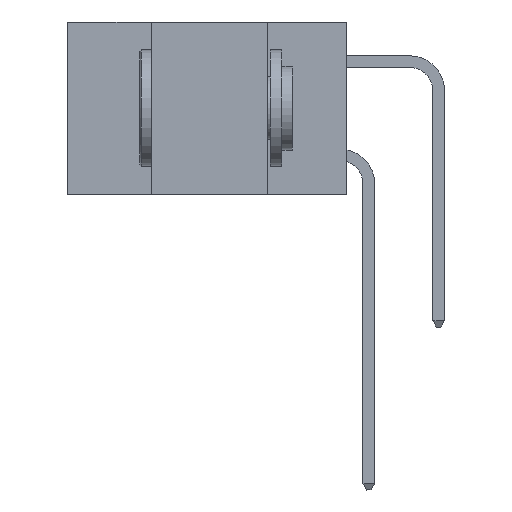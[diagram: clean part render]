
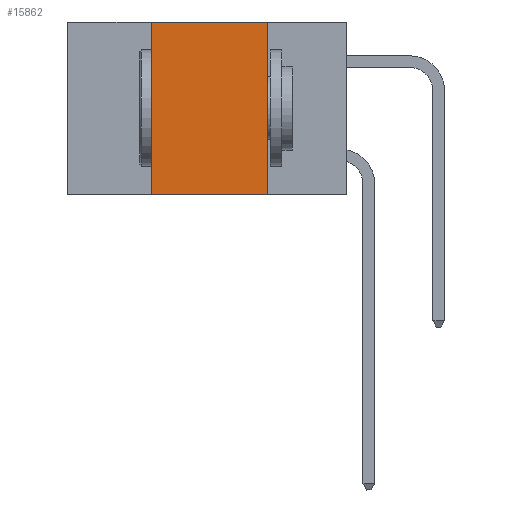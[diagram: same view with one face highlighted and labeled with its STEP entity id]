
A CAD part, left-side view. The second image highlights one B-rep face of the part: STEP entity #15862.
In plain terms, the highlighted planar face has unit normal (-1, 0, 0).
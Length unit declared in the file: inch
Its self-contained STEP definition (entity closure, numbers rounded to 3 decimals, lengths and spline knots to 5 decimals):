
#736 = EDGE_LOOP ( 'NONE', ( #25072, #14019, #37678, #6269 ) ) ;
#1082 = VERTEX_POINT ( 'NONE', #15714 ) ;
#1571 = VERTEX_POINT ( 'NONE', #8951 ) ;
#5653 = PLANE ( 'NONE',  #16178 ) ;
#6269 = ORIENTED_EDGE ( 'NONE', *, *, #40783, .T. ) ;
#6844 = VERTEX_POINT ( 'NONE', #40842 ) ;
#7020 = VECTOR ( 'NONE', #7798, 39.37008 ) ;
#7798 = DIRECTION ( 'NONE',  ( 0., -1., 0. ) ) ;
#8951 = CARTESIAN_POINT ( 'NONE',  ( 0., 0.42, -0.37 ) ) ;
#9311 = DIRECTION ( 'NONE',  ( 0., -1., 0. ) ) ;
#10511 = CARTESIAN_POINT ( 'NONE',  ( 0., 0.6, 0. ) ) ;
#11087 = LINE ( 'NONE', #10511, #7020 ) ;
#11624 = EDGE_CURVE ( 'NONE', #1571, #31572, #41164, .T. ) ;
#14019 = ORIENTED_EDGE ( 'NONE', *, *, #26578, .F. ) ;
#14582 = EDGE_CURVE ( 'NONE', #6844, #1082, #19150, .T. ) ;
#15714 = CARTESIAN_POINT ( 'NONE',  ( 0., 0.17, -0.37 ) ) ;
#15862 = ADVANCED_FACE ( 'NONE', ( #41789 ), #5653, .F. ) ;
#16178 = AXIS2_PLACEMENT_3D ( 'NONE', #28473, #18866, #37911 ) ;
#17213 = LINE ( 'NONE', #19111, #40943 ) ;
#18866 = DIRECTION ( 'NONE',  ( 1., 0., 0. ) ) ;
#19111 = CARTESIAN_POINT ( 'NONE',  ( 0., 0.6, -0.37 ) ) ;
#19150 = LINE ( 'NONE', #24515, #32268 ) ;
#21413 = DIRECTION ( 'NONE',  ( 0., 0., -1. ) ) ;
#23064 = DIRECTION ( 'NONE',  ( 0., 0., 1. ) ) ;
#24515 = CARTESIAN_POINT ( 'NONE',  ( 0., 0.17, 0. ) ) ;
#25072 = ORIENTED_EDGE ( 'NONE', *, *, #14582, .F. ) ;
#26578 = EDGE_CURVE ( 'NONE', #31572, #6844, #11087, .T. ) ;
#26909 = CARTESIAN_POINT ( 'NONE',  ( 0., 0.42, 0. ) ) ;
#28473 = CARTESIAN_POINT ( 'NONE',  ( 0., 0.6, 0. ) ) ;
#31566 = VECTOR ( 'NONE', #23064, 39.37008 ) ;
#31572 = VERTEX_POINT ( 'NONE', #26909 ) ;
#32268 = VECTOR ( 'NONE', #21413, 39.37008 ) ;
#36296 = CARTESIAN_POINT ( 'NONE',  ( 0., 0.42, 0. ) ) ;
#37678 = ORIENTED_EDGE ( 'NONE', *, *, #11624, .F. ) ;
#37911 = DIRECTION ( 'NONE',  ( 0., 0., -1. ) ) ;
#40783 = EDGE_CURVE ( 'NONE', #1571, #1082, #17213, .T. ) ;
#40842 = CARTESIAN_POINT ( 'NONE',  ( 0., 0.17, 0. ) ) ;
#40943 = VECTOR ( 'NONE', #9311, 39.37008 ) ;
#41164 = LINE ( 'NONE', #36296, #31566 ) ;
#41789 = FACE_OUTER_BOUND ( 'NONE', #736, .T. ) ;
